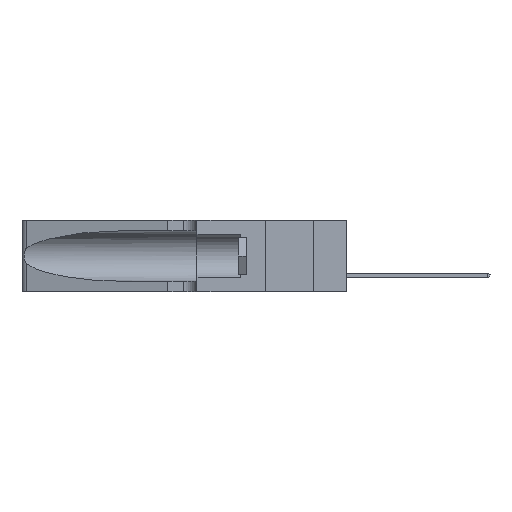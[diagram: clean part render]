
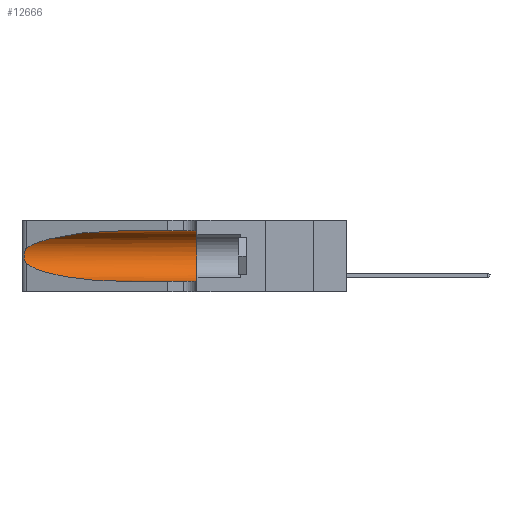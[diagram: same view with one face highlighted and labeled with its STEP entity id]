
A CAD part, left-side view. The second image highlights one B-rep face of the part: STEP entity #12666.
In plain terms, the highlighted cylindrical face has radius 3.308 mm (diameter 6.617 mm), a partial arc.
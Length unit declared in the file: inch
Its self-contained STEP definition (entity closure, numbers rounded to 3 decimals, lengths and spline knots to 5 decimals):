
#322 = ORIENTED_EDGE ( 'NONE', *, *, #10352, .T. ) ;
#2270 = CARTESIAN_POINT ( 'NONE',  ( 0.18966, 0.96281, 0.05475 ) ) ;
#2607 = DIRECTION ( 'NONE',  ( 0., 1., 0. ) ) ;
#2641 = VERTEX_POINT ( 'NONE', #20625 ) ;
#2773 = CARTESIAN_POINT ( 'NONE',  ( 0.1305, 1.61858, 0.31525 ) ) ;
#3858 = CARTESIAN_POINT ( 'NONE',  ( 0.26018, 1.23835, 0.19895 ) ) ;
#4469 = FACE_OUTER_BOUND ( 'NONE', #22460, .T. ) ;
#5439 = LINE ( 'NONE', #18803, #20171 ) ;
#5614 = LINE ( 'NONE', #2773, #6640 ) ;
#5958 = CARTESIAN_POINT ( 'NONE',  ( 0.25639, 1.23184, 0.21858 ) ) ;
#6489 = CARTESIAN_POINT ( 'NONE',  ( 0.1305, 0.72297, 0.05475 ) ) ;
#6640 = VECTOR ( 'NONE', #23798, 39.37008 ) ;
#7465 = CIRCLE ( 'NONE', #14417, 0.13025 ) ;
#7540 = VERTEX_POINT ( 'NONE', #15260 ) ;
#7991 = ORIENTED_EDGE ( 'NONE', *, *, #14820, .F. ) ;
#8206 = VERTEX_POINT ( 'NONE', #13556 ) ;
#8878 = CARTESIAN_POINT ( 'NONE',  ( 0.2373, 1.15595, 0.08982 ) ) ;
#10199 = EDGE_CURVE ( 'NONE', #14336, #8206, #18677, .T. ) ;
#10261 = DIRECTION ( 'NONE',  ( 0., -1., 0. ) ) ;
#10352 = EDGE_CURVE ( 'NONE', #2641, #11370, #5439, .T. ) ;
#10518 = EDGE_CURVE ( 'NONE', #8206, #2641, #26378, .T. ) ;
#10810 = CARTESIAN_POINT ( 'NONE',  ( 0.25555, 1.22993, 0.14849 ) ) ;
#11370 = VERTEX_POINT ( 'NONE', #13603 ) ;
#11493 = CARTESIAN_POINT ( 'NONE',  ( 0.1305, 1.61858, 0.185 ) ) ;
#11683 = CARTESIAN_POINT ( 'NONE',  ( 0.18966, 0.96281, 0.31525 ) ) ;
#12203 = CARTESIAN_POINT ( 'NONE',  ( 0.25854, 1.2359, 0.20912 ) ) ;
#12578 = EDGE_CURVE ( 'NONE', #21172, #11370, #7465, .T. ) ;
#12666 = ADVANCED_FACE ( 'NONE', ( #4469 ), #14948, .F. ) ;
#12965 = CARTESIAN_POINT ( 'NONE',  ( 0.25487, 1.22718, 0.14631 ) ) ;
#13043 = CARTESIAN_POINT ( 'NONE',  ( 0.25487, 1.22718, 0.22369 ) ) ;
#13342 = ORIENTED_EDGE ( 'NONE', *, *, #18463, .T. ) ;
#13556 = CARTESIAN_POINT ( 'NONE',  ( 0.25487, 1.22718, 0.14631 ) ) ;
#13603 = CARTESIAN_POINT ( 'NONE',  ( 0.1305, 0.35, 0.05475 ) ) ;
#13757 = CARTESIAN_POINT ( 'NONE',  ( 0.25487, 1.22718, 0.22369 ) ) ;
#14336 = VERTEX_POINT ( 'NONE', #13043 ) ;
#14382 = CARTESIAN_POINT ( 'NONE',  ( 0.26017, 1.23833, 0.17102 ) ) ;
#14417 = AXIS2_PLACEMENT_3D ( 'NONE', #25522, #2607, #23974 ) ;
#14820 = EDGE_CURVE ( 'NONE', #7540, #21172, #5614, .T. ) ;
#14948 = CYLINDRICAL_SURFACE ( 'NONE', #25952, 0.13025 ) ;
#15006 = CARTESIAN_POINT ( 'NONE',  ( 0.25487, 1.22718, 0.14631 ) ) ;
#15260 = CARTESIAN_POINT ( 'NONE',  ( 0.1305, 0.72297, 0.31525 ) ) ;
#15963 = CARTESIAN_POINT ( 'NONE',  ( 0.25487, 1.22718, 0.22369 ) ) ;
#16186 =( BOUNDED_CURVE ( )  B_SPLINE_CURVE ( 3, ( #26542, #11683, #26261, #15963 ),
 .UNSPECIFIED., .F., .T. ) 
 B_SPLINE_CURVE_WITH_KNOTS ( ( 4, 4 ),
 ( 1.5708, 2.84003 ),
 .UNSPECIFIED. ) 
 CURVE ( )  GEOMETRIC_REPRESENTATION_ITEM ( )  RATIONAL_B_SPLINE_CURVE ( ( 1., 0.87, 0.87, 1. ) ) 
 REPRESENTATION_ITEM ( '' )  );
#17947 = DIRECTION ( 'NONE',  ( 0., 0., -1. ) ) ;
#18463 = EDGE_CURVE ( 'NONE', #7540, #14336, #16186, .T. ) ;
#18567 = CARTESIAN_POINT ( 'NONE',  ( 0.25856, 1.23593, 0.16098 ) ) ;
#18677 = B_SPLINE_CURVE_WITH_KNOTS ( 'NONE', 3,
 ( #13757, #18742, #5958, #24594, #12203, #3858, #24762, #26903, #14382, #18567, #22765, #25315, #10810, #15006 ),
 .UNSPECIFIED., .F., .F.,
 ( 4, 2, 2, 2, 2, 2, 4 ),
 ( 0., 0.00027, 0.00053, 0.00107, 0.0016, 0.00187, 0.00214 ),
 .UNSPECIFIED. ) ;
#18742 = CARTESIAN_POINT ( 'NONE',  ( 0.25555, 1.22994, 0.2215 ) ) ;
#18803 = CARTESIAN_POINT ( 'NONE',  ( 0.1305, 1.61858, 0.05475 ) ) ;
#18830 = ORIENTED_EDGE ( 'NONE', *, *, #10199, .T. ) ;
#20171 = VECTOR ( 'NONE', #10261, 39.37008 ) ;
#20625 = CARTESIAN_POINT ( 'NONE',  ( 0.1305, 0.72297, 0.05475 ) ) ;
#21172 = VERTEX_POINT ( 'NONE', #25684 ) ;
#21977 = DIRECTION ( 'NONE',  ( 0., -1., 0. ) ) ;
#22460 = EDGE_LOOP ( 'NONE', ( #13342, #18830, #22552, #322, #25002, #7991 ) ) ;
#22552 = ORIENTED_EDGE ( 'NONE', *, *, #10518, .T. ) ;
#22765 = CARTESIAN_POINT ( 'NONE',  ( 0.25789, 1.23486, 0.15765 ) ) ;
#23798 = DIRECTION ( 'NONE',  ( 0., -1., 0. ) ) ;
#23974 = DIRECTION ( 'NONE',  ( 0., 0., 1. ) ) ;
#24594 = CARTESIAN_POINT ( 'NONE',  ( 0.25787, 1.23484, 0.2124 ) ) ;
#24762 = CARTESIAN_POINT ( 'NONE',  ( 0.26075, 1.23896, 0.19203 ) ) ;
#25002 = ORIENTED_EDGE ( 'NONE', *, *, #12578, .F. ) ;
#25315 = CARTESIAN_POINT ( 'NONE',  ( 0.25639, 1.23186, 0.15144 ) ) ;
#25522 = CARTESIAN_POINT ( 'NONE',  ( 0.1305, 0.35, 0.185 ) ) ;
#25684 = CARTESIAN_POINT ( 'NONE',  ( 0.1305, 0.35, 0.31525 ) ) ;
#25952 = AXIS2_PLACEMENT_3D ( 'NONE', #11493, #21977, #17947 ) ;
#26261 = CARTESIAN_POINT ( 'NONE',  ( 0.2373, 1.15595, 0.28018 ) ) ;
#26378 =( BOUNDED_CURVE ( )  B_SPLINE_CURVE ( 3, ( #12965, #8878, #2270, #6489 ),
 .UNSPECIFIED., .F., .T. ) 
 B_SPLINE_CURVE_WITH_KNOTS ( ( 4, 4 ),
 ( 3.44316, 4.71239 ),
 .UNSPECIFIED. ) 
 CURVE ( )  GEOMETRIC_REPRESENTATION_ITEM ( )  RATIONAL_B_SPLINE_CURVE ( ( 1., 0.87, 0.87, 1. ) ) 
 REPRESENTATION_ITEM ( '' )  );
#26542 = CARTESIAN_POINT ( 'NONE',  ( 0.1305, 0.72297, 0.31525 ) ) ;
#26903 = CARTESIAN_POINT ( 'NONE',  ( 0.26075, 1.23896, 0.178 ) ) ;
